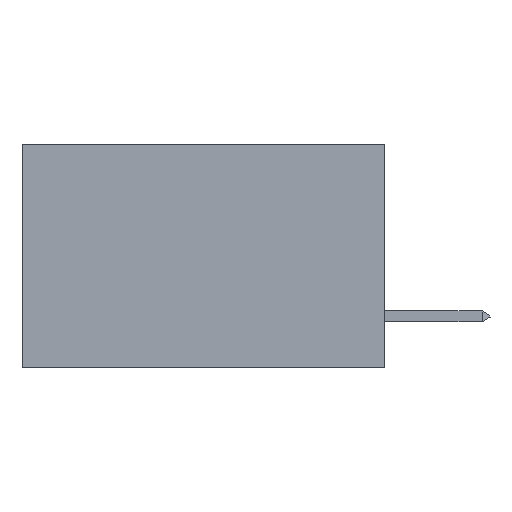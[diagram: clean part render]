
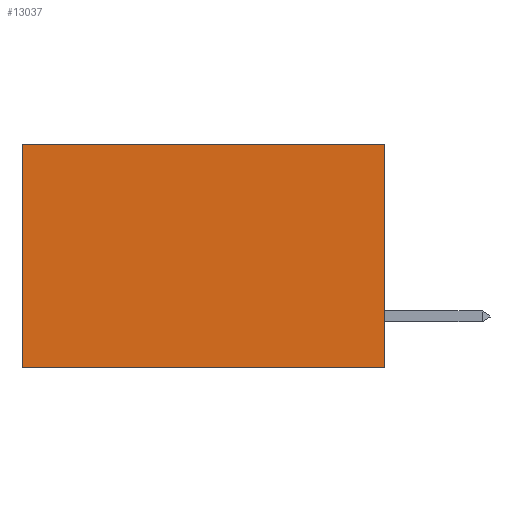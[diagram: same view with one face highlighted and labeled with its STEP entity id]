
A CAD part, left-side view. The second image highlights one B-rep face of the part: STEP entity #13037.
In plain terms, the highlighted planar face has unit normal (-1, 0, 0).
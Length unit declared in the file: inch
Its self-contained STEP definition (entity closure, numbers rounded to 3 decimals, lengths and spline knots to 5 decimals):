
#34 = CARTESIAN_POINT ( 'NONE',  ( 0.2875, 0., 0. ) ) ;
#59 = EDGE_CURVE ( 'NONE', #25309, #21744, #9388, .T. ) ;
#333 = VECTOR ( 'NONE', #11977, 39.37008 ) ;
#486 = DIRECTION ( 'NONE',  ( 0., 1., 0. ) ) ;
#936 = CARTESIAN_POINT ( 'NONE',  ( 0.2875, 0.6, 0. ) ) ;
#1055 = VECTOR ( 'NONE', #486, 39.37008 ) ;
#1105 = CARTESIAN_POINT ( 'NONE',  ( 0.2875, 0.6, 0. ) ) ;
#1405 = DIRECTION ( 'NONE',  ( 1., 0., 0. ) ) ;
#3415 = CARTESIAN_POINT ( 'NONE',  ( 0.2875, 0., 0. ) ) ;
#4740 = DIRECTION ( 'NONE',  ( 0., 0., -1. ) ) ;
#5322 = DIRECTION ( 'NONE',  ( 0., 0., -1. ) ) ;
#7737 = EDGE_CURVE ( 'NONE', #21744, #8070, #19464, .T. ) ;
#8070 = VERTEX_POINT ( 'NONE', #24495 ) ;
#9073 = FACE_OUTER_BOUND ( 'NONE', #11868, .T. ) ;
#9214 = LINE ( 'NONE', #9661, #333 ) ;
#9388 = LINE ( 'NONE', #34, #23384 ) ;
#9661 = CARTESIAN_POINT ( 'NONE',  ( 0.2875, 0., 0. ) ) ;
#11096 = VECTOR ( 'NONE', #5322, 39.37008 ) ;
#11133 = ORIENTED_EDGE ( 'NONE', *, *, #7737, .F. ) ;
#11868 = EDGE_LOOP ( 'NONE', ( #23404, #11133, #26059, #27934 ) ) ;
#11977 = DIRECTION ( 'NONE',  ( 0., 1., 0. ) ) ;
#12257 = PLANE ( 'NONE',  #28124 ) ;
#13037 = ADVANCED_FACE ( 'NONE', ( #9073 ), #12257, .F. ) ;
#13414 = EDGE_CURVE ( 'NONE', #25981, #8070, #24787, .T. ) ;
#14167 = DIRECTION ( 'NONE',  ( 0., 0., -1. ) ) ;
#17856 = CARTESIAN_POINT ( 'NONE',  ( 0.2875, 0., 0. ) ) ;
#18237 = EDGE_CURVE ( 'NONE', #25309, #25981, #9214, .T. ) ;
#19464 = LINE ( 'NONE', #26903, #1055 ) ;
#21744 = VERTEX_POINT ( 'NONE', #22107 ) ;
#22107 = CARTESIAN_POINT ( 'NONE',  ( 0.2875, 0., -0.37 ) ) ;
#23384 = VECTOR ( 'NONE', #4740, 39.37008 ) ;
#23404 = ORIENTED_EDGE ( 'NONE', *, *, #13414, .T. ) ;
#24495 = CARTESIAN_POINT ( 'NONE',  ( 0.2875, 0.6, -0.37 ) ) ;
#24787 = LINE ( 'NONE', #936, #11096 ) ;
#25309 = VERTEX_POINT ( 'NONE', #17856 ) ;
#25981 = VERTEX_POINT ( 'NONE', #1105 ) ;
#26059 = ORIENTED_EDGE ( 'NONE', *, *, #59, .F. ) ;
#26903 = CARTESIAN_POINT ( 'NONE',  ( 0.2875, 0., -0.37 ) ) ;
#27934 = ORIENTED_EDGE ( 'NONE', *, *, #18237, .T. ) ;
#28124 = AXIS2_PLACEMENT_3D ( 'NONE', #3415, #1405, #14167 ) ;
